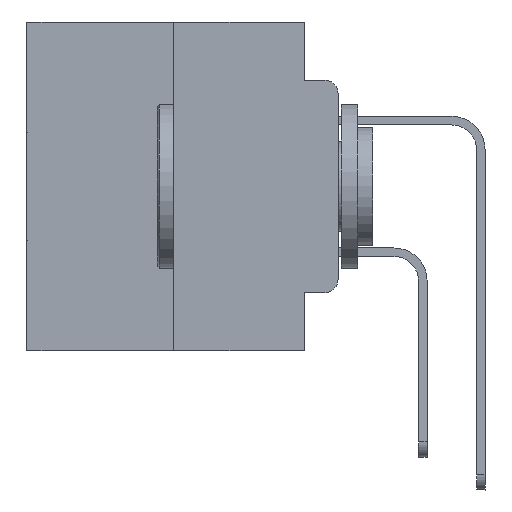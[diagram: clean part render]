
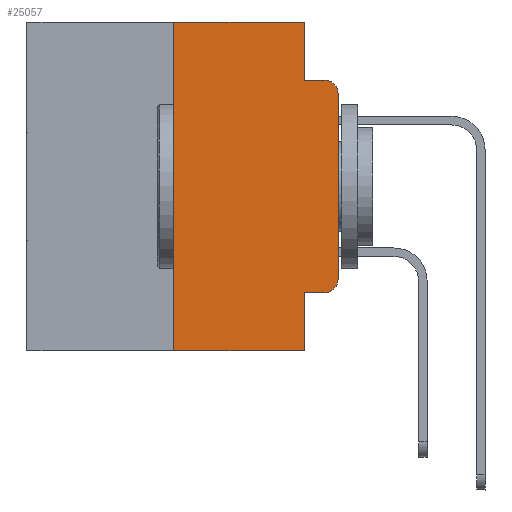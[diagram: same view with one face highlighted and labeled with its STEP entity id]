
A CAD part, left-side view. The second image highlights one B-rep face of the part: STEP entity #25057.
In plain terms, the highlighted planar face has unit normal (-1, 0, 0).
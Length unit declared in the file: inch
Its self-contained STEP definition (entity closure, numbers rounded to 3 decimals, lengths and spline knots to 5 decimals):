
#116 = CARTESIAN_POINT ( 'NONE',  ( 0., 0.02, -0.4115 ) ) ;
#340 = VERTEX_POINT ( 'NONE', #19215 ) ;
#1428 = ORIENTED_EDGE ( 'NONE', *, *, #12180, .F. ) ;
#1637 = DIRECTION ( 'NONE',  ( 0., 0., -1. ) ) ;
#2092 = DIRECTION ( 'NONE',  ( 0., 0., 1. ) ) ;
#2381 = DIRECTION ( 'NONE',  ( 0., 0., -1. ) ) ;
#2566 = EDGE_CURVE ( 'NONE', #340, #16976, #5192, .T. ) ;
#2678 = FACE_OUTER_BOUND ( 'NONE', #17841, .T. ) ;
#2753 = CARTESIAN_POINT ( 'NONE',  ( 0., 0.473, -0.5 ) ) ;
#2970 = DIRECTION ( 'NONE',  ( 0., 0., -1. ) ) ;
#3423 = EDGE_CURVE ( 'NONE', #11823, #16976, #18299, .T. ) ;
#3551 = ORIENTED_EDGE ( 'NONE', *, *, #22920, .T. ) ;
#4599 = CARTESIAN_POINT ( 'NONE',  ( 0., 0.051, -0.5 ) ) ;
#4705 = ORIENTED_EDGE ( 'NONE', *, *, #3423, .F. ) ;
#5030 = CARTESIAN_POINT ( 'NONE',  ( 0., 0.051, -0.4115 ) ) ;
#5192 = LINE ( 'NONE', #2753, #23098 ) ;
#5209 = VECTOR ( 'NONE', #11046, 39.37008 ) ;
#5850 = CARTESIAN_POINT ( 'NONE',  ( 0., 0.25, 0. ) ) ;
#5950 = CARTESIAN_POINT ( 'NONE',  ( 0., 0.051, -0.0885 ) ) ;
#6493 = CARTESIAN_POINT ( 'NONE',  ( 0., 0.051, 0. ) ) ;
#6506 = DIRECTION ( 'NONE',  ( 0., -1., 0. ) ) ;
#6800 = CARTESIAN_POINT ( 'NONE',  ( 0., 0.051, 0. ) ) ;
#6882 = LINE ( 'NONE', #29736, #26967 ) ;
#7154 = VECTOR ( 'NONE', #6506, 39.37008 ) ;
#7546 = PLANE ( 'NONE',  #8840 ) ;
#7610 = LINE ( 'NONE', #5030, #17458 ) ;
#7918 = AXIS2_PLACEMENT_3D ( 'NONE', #17357, #10397, #2970 ) ;
#8632 = ORIENTED_EDGE ( 'NONE', *, *, #2566, .T. ) ;
#8705 = DIRECTION ( 'NONE',  ( 0., 0., 1. ) ) ;
#8840 = AXIS2_PLACEMENT_3D ( 'NONE', #16762, #21174, #2381 ) ;
#9263 = CARTESIAN_POINT ( 'NONE',  ( 0., 0.051, -0.4115 ) ) ;
#9594 = DIRECTION ( 'NONE',  ( 0., -1., 0. ) ) ;
#9631 = EDGE_CURVE ( 'NONE', #16005, #15626, #27087, .T. ) ;
#10397 = DIRECTION ( 'NONE',  ( -1., 0., 0. ) ) ;
#11046 = DIRECTION ( 'NONE',  ( 0., 0., -1. ) ) ;
#11208 = CARTESIAN_POINT ( 'NONE',  ( 0., 0.25, 0. ) ) ;
#11405 = VERTEX_POINT ( 'NONE', #17814 ) ;
#11823 = VERTEX_POINT ( 'NONE', #9263 ) ;
#12054 = DIRECTION ( 'NONE',  ( -1., 0., 0. ) ) ;
#12180 = EDGE_CURVE ( 'NONE', #21621, #16005, #18466, .T. ) ;
#12345 = DIRECTION ( 'NONE',  ( 0., 0., -1. ) ) ;
#13153 = VERTEX_POINT ( 'NONE', #13692 ) ;
#13692 = CARTESIAN_POINT ( 'NONE',  ( 0., 0., -0.3915 ) ) ;
#13733 = ORIENTED_EDGE ( 'NONE', *, *, #9631, .F. ) ;
#14984 = EDGE_CURVE ( 'NONE', #340, #21621, #23298, .T. ) ;
#15626 = VERTEX_POINT ( 'NONE', #5950 ) ;
#16005 = VERTEX_POINT ( 'NONE', #21369 ) ;
#16762 = CARTESIAN_POINT ( 'NONE',  ( 0., 0.473, 0. ) ) ;
#16901 = ORIENTED_EDGE ( 'NONE', *, *, #23783, .T. ) ;
#16976 = VERTEX_POINT ( 'NONE', #4599 ) ;
#17357 = CARTESIAN_POINT ( 'NONE',  ( 0., 0.02, -0.3915 ) ) ;
#17458 = VECTOR ( 'NONE', #27898, 39.37008 ) ;
#17800 = LINE ( 'NONE', #21903, #23697 ) ;
#17814 = CARTESIAN_POINT ( 'NONE',  ( 0., 0., -0.1085 ) ) ;
#17841 = EDGE_LOOP ( 'NONE', ( #24590, #16901, #28208, #13733, #1428, #25462, #8632, #4705, #3551, #25606 ) ) ;
#18257 = VERTEX_POINT ( 'NONE', #116 ) ;
#18299 = LINE ( 'NONE', #6800, #22308 ) ;
#18466 = LINE ( 'NONE', #27694, #7154 ) ;
#18944 = AXIS2_PLACEMENT_3D ( 'NONE', #19148, #12054, #12345 ) ;
#19148 = CARTESIAN_POINT ( 'NONE',  ( 0., 0.02, -0.1085 ) ) ;
#19215 = CARTESIAN_POINT ( 'NONE',  ( 0., 0.25, -0.5 ) ) ;
#19417 = CIRCLE ( 'NONE', #18944, 0.02 ) ;
#20463 = EDGE_CURVE ( 'NONE', #13153, #11405, #6882, .T. ) ;
#21174 = DIRECTION ( 'NONE',  ( 1., 0., 0. ) ) ;
#21369 = CARTESIAN_POINT ( 'NONE',  ( 0., 0.051, 0. ) ) ;
#21621 = VERTEX_POINT ( 'NONE', #5850 ) ;
#21903 = CARTESIAN_POINT ( 'NONE',  ( 0., 0.051, -0.0885 ) ) ;
#22239 = EDGE_CURVE ( 'NONE', #15626, #25731, #17800, .T. ) ;
#22308 = VECTOR ( 'NONE', #1637, 39.37008 ) ;
#22688 = VECTOR ( 'NONE', #2092, 39.37008 ) ;
#22920 = EDGE_CURVE ( 'NONE', #11823, #18257, #7610, .T. ) ;
#23098 = VECTOR ( 'NONE', #9594, 39.37008 ) ;
#23298 = LINE ( 'NONE', #11208, #22688 ) ;
#23697 = VECTOR ( 'NONE', #24607, 39.37008 ) ;
#23783 = EDGE_CURVE ( 'NONE', #11405, #25731, #19417, .T. ) ;
#24590 = ORIENTED_EDGE ( 'NONE', *, *, #20463, .T. ) ;
#24607 = DIRECTION ( 'NONE',  ( 0., -1., 0. ) ) ;
#25057 = ADVANCED_FACE ( 'NONE', ( #2678 ), #7546, .F. ) ;
#25462 = ORIENTED_EDGE ( 'NONE', *, *, #14984, .F. ) ;
#25606 = ORIENTED_EDGE ( 'NONE', *, *, #27287, .T. ) ;
#25731 = VERTEX_POINT ( 'NONE', #26979 ) ;
#26769 = CIRCLE ( 'NONE', #7918, 0.02 ) ;
#26967 = VECTOR ( 'NONE', #8705, 39.37008 ) ;
#26979 = CARTESIAN_POINT ( 'NONE',  ( 0., 0.02, -0.0885 ) ) ;
#27087 = LINE ( 'NONE', #6493, #5209 ) ;
#27287 = EDGE_CURVE ( 'NONE', #18257, #13153, #26769, .T. ) ;
#27694 = CARTESIAN_POINT ( 'NONE',  ( 0., 0.473, 0. ) ) ;
#27898 = DIRECTION ( 'NONE',  ( 0., -1., 0. ) ) ;
#28208 = ORIENTED_EDGE ( 'NONE', *, *, #22239, .F. ) ;
#29736 = CARTESIAN_POINT ( 'NONE',  ( 0., 0., 0. ) ) ;
